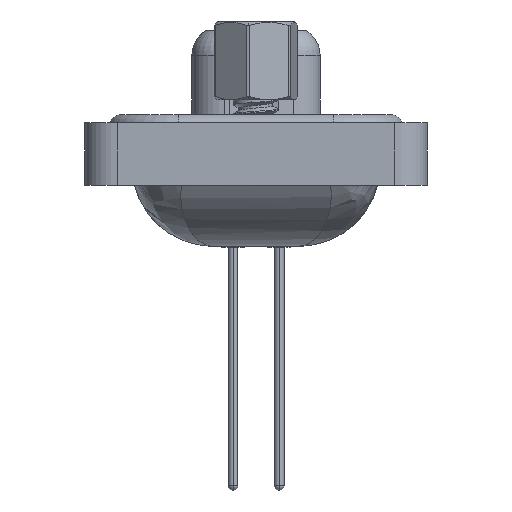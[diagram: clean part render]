
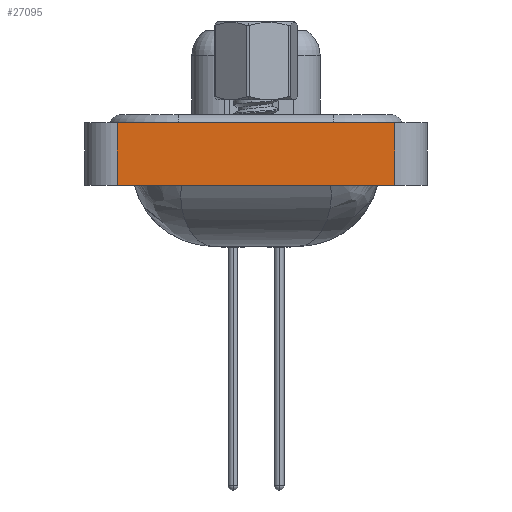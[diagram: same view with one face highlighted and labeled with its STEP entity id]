
A CAD part, left-side view. The second image highlights one B-rep face of the part: STEP entity #27095.
In plain terms, the highlighted planar face has unit normal (-1, 0, 0).
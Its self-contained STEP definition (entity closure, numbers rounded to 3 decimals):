
#425 = VECTOR ( 'NONE', #11203, 1000. ) ;
#5249 = VECTOR ( 'NONE', #19972, 1000. ) ;
#6130 = CARTESIAN_POINT ( 'NONE',  ( -7.15, -8.55, -3.35 ) ) ;
#6528 = EDGE_LOOP ( 'NONE', ( #11954, #20581, #27452, #19218 ) ) ;
#7426 = EDGE_CURVE ( 'NONE', #25320, #32753, #21880, .T. ) ;
#11046 = AXIS2_PLACEMENT_3D ( 'NONE', #6130, #29555, #32537 ) ;
#11203 = DIRECTION ( 'NONE',  ( 0., -1., 0. ) ) ;
#11954 = ORIENTED_EDGE ( 'NONE', *, *, #33619, .T. ) ;
#12556 = LINE ( 'NONE', #31327, #18921 ) ;
#13218 = EDGE_CURVE ( 'NONE', #25320, #17933, #12556, .T. ) ;
#14724 = CARTESIAN_POINT ( 'NONE',  ( -7.15, -8.55, -3.35 ) ) ;
#15530 = DIRECTION ( 'NONE',  ( 0., 0., 1. ) ) ;
#16239 = DIRECTION ( 'NONE',  ( 0., -1., 0. ) ) ;
#16918 = VERTEX_POINT ( 'NONE', #32063 ) ;
#17415 = CARTESIAN_POINT ( 'NONE',  ( -7.15, 8.55, 0.5 ) ) ;
#17933 = VERTEX_POINT ( 'NONE', #17415 ) ;
#18663 = EDGE_CURVE ( 'NONE', #17933, #16918, #21309, .T. ) ;
#18921 = VECTOR ( 'NONE', #15530, 1000. ) ;
#19126 = VECTOR ( 'NONE', #16239, 1000. ) ;
#19218 = ORIENTED_EDGE ( 'NONE', *, *, #7426, .T. ) ;
#19862 = CARTESIAN_POINT ( 'NONE',  ( -7.15, 8.55, -3.35 ) ) ;
#19972 = DIRECTION ( 'NONE',  ( 0., 0., 1. ) ) ;
#20138 = FACE_OUTER_BOUND ( 'NONE', #6528, .T. ) ;
#20581 = ORIENTED_EDGE ( 'NONE', *, *, #18663, .F. ) ;
#21309 = LINE ( 'NONE', #24647, #19126 ) ;
#21880 = LINE ( 'NONE', #24333, #425 ) ;
#22954 = LINE ( 'NONE', #14724, #5249 ) ;
#23705 = CARTESIAN_POINT ( 'NONE',  ( -7.15, -8.55, -3.35 ) ) ;
#24333 = CARTESIAN_POINT ( 'NONE',  ( -7.15, -8.55, -3.35 ) ) ;
#24647 = CARTESIAN_POINT ( 'NONE',  ( -7.15, -8.55, 0.5 ) ) ;
#25320 = VERTEX_POINT ( 'NONE', #19862 ) ;
#27095 = ADVANCED_FACE ( 'NONE', ( #20138 ), #30157, .T. ) ;
#27452 = ORIENTED_EDGE ( 'NONE', *, *, #13218, .F. ) ;
#29555 = DIRECTION ( 'NONE',  ( -1., 0., 0. ) ) ;
#30157 = PLANE ( 'NONE',  #11046 ) ;
#31327 = CARTESIAN_POINT ( 'NONE',  ( -7.15, 8.55, -3.35 ) ) ;
#32063 = CARTESIAN_POINT ( 'NONE',  ( -7.15, -8.55, 0.5 ) ) ;
#32537 = DIRECTION ( 'NONE',  ( 0., 0., 1. ) ) ;
#32753 = VERTEX_POINT ( 'NONE', #23705 ) ;
#33619 = EDGE_CURVE ( 'NONE', #32753, #16918, #22954, .T. ) ;
